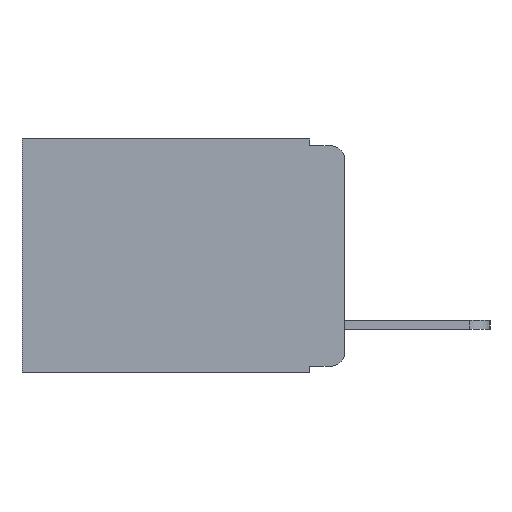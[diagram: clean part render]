
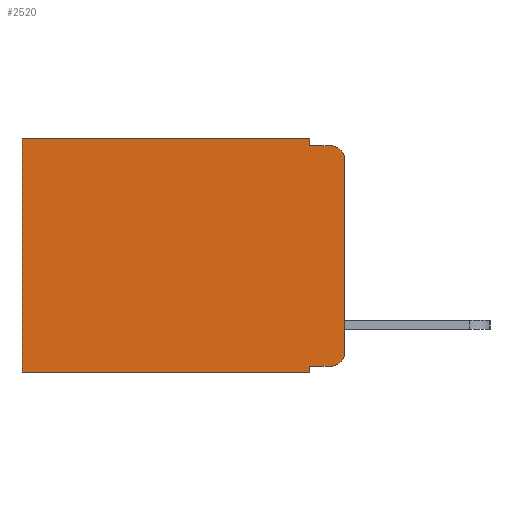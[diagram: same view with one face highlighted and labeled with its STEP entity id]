
A CAD part, left-side view. The second image highlights one B-rep face of the part: STEP entity #2520.
In plain terms, the highlighted planar face has unit normal (-1, 0, 0).
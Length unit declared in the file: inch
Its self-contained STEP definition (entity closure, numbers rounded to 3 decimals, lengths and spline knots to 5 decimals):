
#19 = LINE ( 'NONE', #4712, #2111 ) ;
#23 = EDGE_CURVE ( 'NONE', #2639, #11114, #8143, .T. ) ;
#198 = VERTEX_POINT ( 'NONE', #6459 ) ;
#199 = EDGE_CURVE ( 'NONE', #9150, #11114, #3966, .T. ) ;
#262 = EDGE_CURVE ( 'NONE', #12076, #1453, #3873, .T. ) ;
#814 = EDGE_CURVE ( 'NONE', #6790, #9150, #19, .T. ) ;
#1169 = VECTOR ( 'NONE', #11843, 39.37008 ) ;
#1453 = VERTEX_POINT ( 'NONE', #10324 ) ;
#1924 = VERTEX_POINT ( 'NONE', #10792 ) ;
#1977 = DIRECTION ( 'NONE',  ( 0., 0., -1. ) ) ;
#2014 = EDGE_CURVE ( 'NONE', #2639, #198, #4953, .T. ) ;
#2111 = VECTOR ( 'NONE', #8800, 39.37008 ) ;
#2520 = ADVANCED_FACE ( 'NONE', ( #10936 ), #5524, .F. ) ;
#2639 = VERTEX_POINT ( 'NONE', #5330 ) ;
#3239 = VERTEX_POINT ( 'NONE', #8536 ) ;
#3530 = LINE ( 'NONE', #11236, #6853 ) ;
#3873 = LINE ( 'NONE', #10983, #6035 ) ;
#3966 = CIRCLE ( 'NONE', #8498, 0.02 ) ;
#3984 = DIRECTION ( 'NONE',  ( 0., 1., 0. ) ) ;
#4712 = CARTESIAN_POINT ( 'NONE',  ( 0.298, 0.051, -0.333 ) ) ;
#4953 = CIRCLE ( 'NONE', #5523, 0.02 ) ;
#5330 = CARTESIAN_POINT ( 'NONE',  ( 0.298, 0., -0.03 ) ) ;
#5523 = AXIS2_PLACEMENT_3D ( 'NONE', #9410, #9397, #9127 ) ;
#5524 = PLANE ( 'NONE',  #9417 ) ;
#5576 = ORIENTED_EDGE ( 'NONE', *, *, #6513, .F. ) ;
#6006 = CARTESIAN_POINT ( 'NONE',  ( 0.298, 0.473, 0. ) ) ;
#6035 = VECTOR ( 'NONE', #9898, 39.37008 ) ;
#6091 = CARTESIAN_POINT ( 'NONE',  ( 0.298, 0.051, 0. ) ) ;
#6147 = CARTESIAN_POINT ( 'NONE',  ( 0.298, 0.051, -0.333 ) ) ;
#6269 = DIRECTION ( 'NONE',  ( 0., 0., -1. ) ) ;
#6459 = CARTESIAN_POINT ( 'NONE',  ( 0.298, 0.02, -0.01 ) ) ;
#6513 = EDGE_CURVE ( 'NONE', #9654, #198, #3530, .T. ) ;
#6606 = DIRECTION ( 'NONE',  ( 0., 0., -1. ) ) ;
#6648 = VECTOR ( 'NONE', #9100, 39.37008 ) ;
#6790 = VERTEX_POINT ( 'NONE', #6147 ) ;
#6853 = VECTOR ( 'NONE', #11844, 39.37008 ) ;
#7119 = VECTOR ( 'NONE', #6606, 39.37008 ) ;
#7214 = LINE ( 'NONE', #10999, #9426 ) ;
#7466 = LINE ( 'NONE', #10576, #6648 ) ;
#7524 = CARTESIAN_POINT ( 'NONE',  ( 0.298, 0.051, 0. ) ) ;
#8115 = EDGE_CURVE ( 'NONE', #1924, #9654, #10954, .T. ) ;
#8143 = LINE ( 'NONE', #8722, #7119 ) ;
#8156 = CARTESIAN_POINT ( 'NONE',  ( 0.298, 0.02, -0.333 ) ) ;
#8216 = ORIENTED_EDGE ( 'NONE', *, *, #11052, .F. ) ;
#8383 = ORIENTED_EDGE ( 'NONE', *, *, #814, .T. ) ;
#8460 = ORIENTED_EDGE ( 'NONE', *, *, #199, .T. ) ;
#8493 = ORIENTED_EDGE ( 'NONE', *, *, #262, .T. ) ;
#8498 = AXIS2_PLACEMENT_3D ( 'NONE', #11688, #11493, #11503 ) ;
#8510 = ORIENTED_EDGE ( 'NONE', *, *, #10861, .F. ) ;
#8536 = CARTESIAN_POINT ( 'NONE',  ( 0.298, 0.051, -0.343 ) ) ;
#8571 = CARTESIAN_POINT ( 'NONE',  ( 0.298, 0.051, -0.01 ) ) ;
#8602 = CARTESIAN_POINT ( 'NONE',  ( 0.298, 0., -0.313 ) ) ;
#8722 = CARTESIAN_POINT ( 'NONE',  ( 0.298, 0., 0. ) ) ;
#8800 = DIRECTION ( 'NONE',  ( 0., -1., 0. ) ) ;
#9100 = DIRECTION ( 'NONE',  ( 0., 1., 0. ) ) ;
#9127 = DIRECTION ( 'NONE',  ( 0., 0., -1. ) ) ;
#9135 = ORIENTED_EDGE ( 'NONE', *, *, #2014, .T. ) ;
#9150 = VERTEX_POINT ( 'NONE', #8156 ) ;
#9397 = DIRECTION ( 'NONE',  ( -1., 0., 0. ) ) ;
#9410 = CARTESIAN_POINT ( 'NONE',  ( 0.298, 0.02, -0.03 ) ) ;
#9417 = AXIS2_PLACEMENT_3D ( 'NONE', #11144, #11508, #6269 ) ;
#9426 = VECTOR ( 'NONE', #3984, 39.37008 ) ;
#9547 = EDGE_LOOP ( 'NONE', ( #11513, #9135, #5576, #11715, #11889, #8493, #8510, #8216, #8383, #8460 ) ) ;
#9654 = VERTEX_POINT ( 'NONE', #8571 ) ;
#9898 = DIRECTION ( 'NONE',  ( 0., 0., -1. ) ) ;
#10069 = VECTOR ( 'NONE', #1977, 39.37008 ) ;
#10324 = CARTESIAN_POINT ( 'NONE',  ( 0.298, 0.473, -0.343 ) ) ;
#10576 = CARTESIAN_POINT ( 'NONE',  ( 0.298, 0., -0.343 ) ) ;
#10792 = CARTESIAN_POINT ( 'NONE',  ( 0.298, 0.051, 0. ) ) ;
#10861 = EDGE_CURVE ( 'NONE', #3239, #1453, #7466, .T. ) ;
#10936 = FACE_OUTER_BOUND ( 'NONE', #9547, .T. ) ;
#10954 = LINE ( 'NONE', #6091, #10069 ) ;
#10983 = CARTESIAN_POINT ( 'NONE',  ( 0.298, 0.473, 0. ) ) ;
#10999 = CARTESIAN_POINT ( 'NONE',  ( 0.298, 0., 0. ) ) ;
#11005 = LINE ( 'NONE', #7524, #1169 ) ;
#11052 = EDGE_CURVE ( 'NONE', #6790, #3239, #11005, .T. ) ;
#11114 = VERTEX_POINT ( 'NONE', #8602 ) ;
#11144 = CARTESIAN_POINT ( 'NONE',  ( 0.298, 0., 0. ) ) ;
#11236 = CARTESIAN_POINT ( 'NONE',  ( 0.298, 0.051, -0.01 ) ) ;
#11493 = DIRECTION ( 'NONE',  ( -1., 0., 0. ) ) ;
#11503 = DIRECTION ( 'NONE',  ( 0., 0., -1. ) ) ;
#11508 = DIRECTION ( 'NONE',  ( 1., 0., 0. ) ) ;
#11513 = ORIENTED_EDGE ( 'NONE', *, *, #23, .F. ) ;
#11688 = CARTESIAN_POINT ( 'NONE',  ( 0.298, 0.02, -0.313 ) ) ;
#11715 = ORIENTED_EDGE ( 'NONE', *, *, #8115, .F. ) ;
#11843 = DIRECTION ( 'NONE',  ( 0., 0., -1. ) ) ;
#11844 = DIRECTION ( 'NONE',  ( 0., -1., 0. ) ) ;
#11889 = ORIENTED_EDGE ( 'NONE', *, *, #12085, .T. ) ;
#12076 = VERTEX_POINT ( 'NONE', #6006 ) ;
#12085 = EDGE_CURVE ( 'NONE', #1924, #12076, #7214, .T. ) ;
